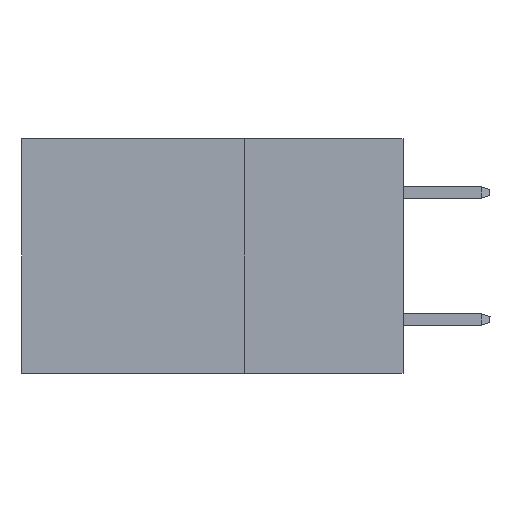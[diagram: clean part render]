
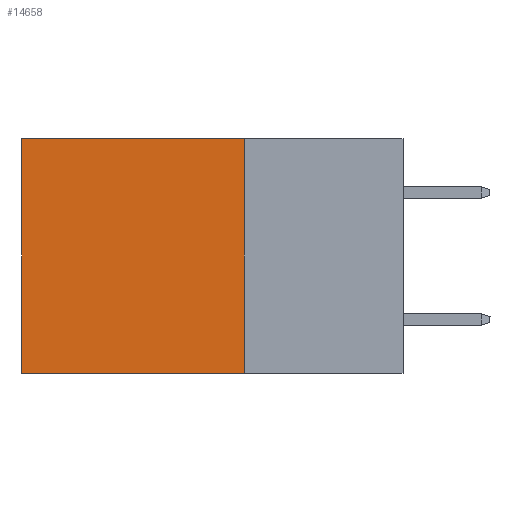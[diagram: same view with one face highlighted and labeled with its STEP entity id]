
A CAD part, left-side view. The second image highlights one B-rep face of the part: STEP entity #14658.
In plain terms, the highlighted planar face has unit normal (-1, 0, 0).
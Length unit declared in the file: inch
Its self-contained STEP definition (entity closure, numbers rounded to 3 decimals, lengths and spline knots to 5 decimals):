
#51 = VERTEX_POINT ( 'NONE', #9289 ) ;
#77 = CARTESIAN_POINT ( 'NONE',  ( 0.2875, 0.25, -0.37 ) ) ;
#177 = ORIENTED_EDGE ( 'NONE', *, *, #12613, .F. ) ;
#1325 = CARTESIAN_POINT ( 'NONE',  ( 0.2875, 0.25, -0.37 ) ) ;
#1784 = VERTEX_POINT ( 'NONE', #13719 ) ;
#2423 = LINE ( 'NONE', #3712, #13393 ) ;
#2543 = CARTESIAN_POINT ( 'NONE',  ( 0.2875, 0.6, -0.37 ) ) ;
#2924 = VECTOR ( 'NONE', #6270, 39.37008 ) ;
#3150 = PLANE ( 'NONE',  #13702 ) ;
#3227 = FACE_OUTER_BOUND ( 'NONE', #6297, .T. ) ;
#3264 = EDGE_CURVE ( 'NONE', #12345, #13041, #7733, .T. ) ;
#3344 = DIRECTION ( 'NONE',  ( 0., 1., 0. ) ) ;
#3701 = EDGE_CURVE ( 'NONE', #1784, #13041, #11047, .T. ) ;
#3702 = ORIENTED_EDGE ( 'NONE', *, *, #10767, .T. ) ;
#3712 = CARTESIAN_POINT ( 'NONE',  ( 0.2875, 0.25, 0. ) ) ;
#3735 = CARTESIAN_POINT ( 'NONE',  ( 0.2875, 0.6, 0. ) ) ;
#4512 = DIRECTION ( 'NONE',  ( 0., 0., -1. ) ) ;
#4580 = DIRECTION ( 'NONE',  ( 0., 0., -1. ) ) ;
#5910 = CARTESIAN_POINT ( 'NONE',  ( 0.2875, 0.25, 0. ) ) ;
#6270 = DIRECTION ( 'NONE',  ( 0., 1., 0. ) ) ;
#6297 = EDGE_LOOP ( 'NONE', ( #11785, #11447, #177, #3702 ) ) ;
#7733 = LINE ( 'NONE', #1325, #2924 ) ;
#9289 = CARTESIAN_POINT ( 'NONE',  ( 0.2875, 0.25, 0. ) ) ;
#9961 = VECTOR ( 'NONE', #15985, 39.37008 ) ;
#10767 = EDGE_CURVE ( 'NONE', #51, #1784, #2423, .T. ) ;
#10771 = CARTESIAN_POINT ( 'NONE',  ( 0.2875, 0.25, 0. ) ) ;
#11047 = LINE ( 'NONE', #3735, #9961 ) ;
#11447 = ORIENTED_EDGE ( 'NONE', *, *, #3264, .F. ) ;
#11785 = ORIENTED_EDGE ( 'NONE', *, *, #3701, .T. ) ;
#12345 = VERTEX_POINT ( 'NONE', #77 ) ;
#12613 = EDGE_CURVE ( 'NONE', #51, #12345, #15635, .T. ) ;
#13041 = VERTEX_POINT ( 'NONE', #2543 ) ;
#13393 = VECTOR ( 'NONE', #3344, 39.37008 ) ;
#13702 = AXIS2_PLACEMENT_3D ( 'NONE', #10771, #15706, #4580 ) ;
#13719 = CARTESIAN_POINT ( 'NONE',  ( 0.2875, 0.6, 0. ) ) ;
#14658 = ADVANCED_FACE ( 'NONE', ( #3227 ), #3150, .F. ) ;
#14929 = VECTOR ( 'NONE', #4512, 39.37008 ) ;
#15635 = LINE ( 'NONE', #5910, #14929 ) ;
#15706 = DIRECTION ( 'NONE',  ( 1., 0., 0. ) ) ;
#15985 = DIRECTION ( 'NONE',  ( 0., 0., -1. ) ) ;
